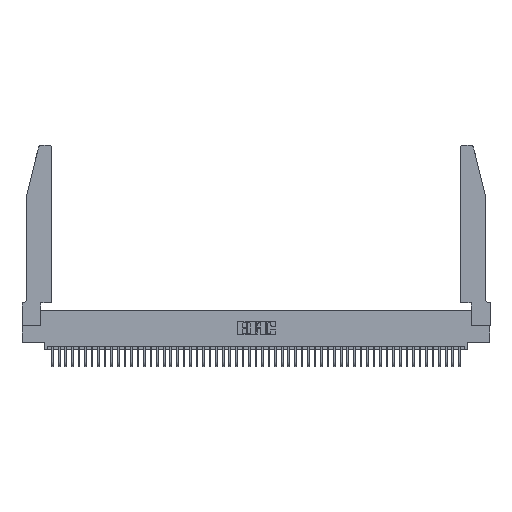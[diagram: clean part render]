
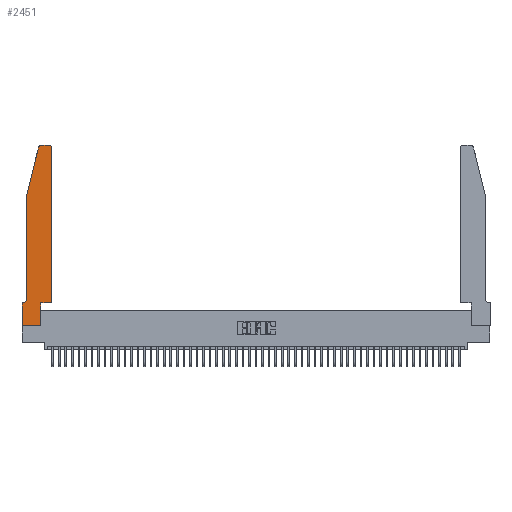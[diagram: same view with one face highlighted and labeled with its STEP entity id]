
A CAD part, top view. The second image highlights one B-rep face of the part: STEP entity #2451.
In plain terms, the highlighted planar face has unit normal (0, 0, 1).
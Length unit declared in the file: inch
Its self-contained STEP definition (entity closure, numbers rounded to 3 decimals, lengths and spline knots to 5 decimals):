
#269 = CARTESIAN_POINT ( 'NONE',  ( 0.0755, 2., 0.37 ) ) ;
#425 = ORIENTED_EDGE ( 'NONE', *, *, #27910, .T. ) ;
#470 = DIRECTION ( 'NONE',  ( 1., 0., 0. ) ) ;
#558 = LINE ( 'NONE', #24356, #9575 ) ;
#656 = EDGE_CURVE ( 'NONE', #18572, #30983, #21931, .T. ) ;
#1385 = DIRECTION ( 'NONE',  ( 0., 1., 0. ) ) ;
#2451 = ADVANCED_FACE ( 'NONE', ( #30536 ), #37271, .T. ) ;
#2888 = DIRECTION ( 'NONE',  ( -1., 0., 0. ) ) ;
#3315 = CARTESIAN_POINT ( 'NONE',  ( 0.2865, 0., 0.37 ) ) ;
#3904 = AXIS2_PLACEMENT_3D ( 'NONE', #21573, #48271, #25416 ) ;
#4101 = CARTESIAN_POINT ( 'NONE',  ( 0.0755, 2., 0.37 ) ) ;
#4486 = EDGE_CURVE ( 'NONE', #43937, #42492, #41733, .T. ) ;
#5169 = CARTESIAN_POINT ( 'NONE',  ( 0.4205, 2.72, 0.37 ) ) ;
#6254 = DIRECTION ( 'NONE',  ( -1., 0., 0. ) ) ;
#6842 = AXIS2_PLACEMENT_3D ( 'NONE', #14297, #18176, #44928 ) ;
#7370 = CARTESIAN_POINT ( 'NONE',  ( 0.25487, 2.72718, 0.37 ) ) ;
#7932 = DIRECTION ( 'NONE',  ( -0.239, -0.971, 0. ) ) ;
#9020 = DIRECTION ( 'NONE',  ( 1., 0., 0. ) ) ;
#9254 = CARTESIAN_POINT ( 'NONE',  ( 0.2865, 0.35, 0.37 ) ) ;
#9575 = VECTOR ( 'NONE', #1385, 39.37008 ) ;
#10505 = LINE ( 'NONE', #15912, #29719 ) ;
#11327 = VECTOR ( 'NONE', #470, 39.37008 ) ;
#12124 = VECTOR ( 'NONE', #2888, 39.37008 ) ;
#13703 = ORIENTED_EDGE ( 'NONE', *, *, #18633, .T. ) ;
#13829 = VECTOR ( 'NONE', #34802, 39.37008 ) ;
#14230 = ORIENTED_EDGE ( 'NONE', *, *, #18502, .T. ) ;
#14297 = CARTESIAN_POINT ( 'NONE',  ( 0., 0.35, 0.37 ) ) ;
#14306 = CIRCLE ( 'NONE', #48393, 0.03 ) ;
#14677 = VERTEX_POINT ( 'NONE', #43139 ) ;
#15912 = CARTESIAN_POINT ( 'NONE',  ( 0.2865, 0.35, 0.37 ) ) ;
#16066 = EDGE_CURVE ( 'NONE', #18029, #41236, #40901, .T. ) ;
#16502 = CARTESIAN_POINT ( 'NONE',  ( 0., 0., 0.37 ) ) ;
#16604 = AXIS2_PLACEMENT_3D ( 'NONE', #44516, #21641, #48350 ) ;
#17129 = ORIENTED_EDGE ( 'NONE', *, *, #16066, .T. ) ;
#17133 = CARTESIAN_POINT ( 'NONE',  ( 0.0055, 0.35, 0.37 ) ) ;
#18029 = VERTEX_POINT ( 'NONE', #43703 ) ;
#18176 = DIRECTION ( 'NONE',  ( 0., 0., 1. ) ) ;
#18502 = EDGE_CURVE ( 'NONE', #46680, #31567, #30557, .T. ) ;
#18572 = VERTEX_POINT ( 'NONE', #23942 ) ;
#18633 = EDGE_CURVE ( 'NONE', #31707, #37220, #14306, .T. ) ;
#19508 = VECTOR ( 'NONE', #7932, 39.37008 ) ;
#20378 = ORIENTED_EDGE ( 'NONE', *, *, #21464, .T. ) ;
#20424 = EDGE_LOOP ( 'NONE', ( #28713, #44259, #20378, #39838, #17129, #42898, #425, #14230, #44186, #38826, #29325, #13703 ) ) ;
#21464 = EDGE_CURVE ( 'NONE', #30983, #14677, #39894, .T. ) ;
#21573 = CARTESIAN_POINT ( 'NONE',  ( 0.284, 2.72, 0.37 ) ) ;
#21641 = DIRECTION ( 'NONE',  ( 0., 0., -1. ) ) ;
#21931 = CIRCLE ( 'NONE', #3904, 0.03 ) ;
#23225 = CARTESIAN_POINT ( 'NONE',  ( 0.4505, 2.72, 0.37 ) ) ;
#23458 = CARTESIAN_POINT ( 'NONE',  ( 0., 0., 0.37 ) ) ;
#23783 = LINE ( 'NONE', #48816, #33989 ) ;
#23942 = CARTESIAN_POINT ( 'NONE',  ( 0.284, 2.75, 0.37 ) ) ;
#24356 = CARTESIAN_POINT ( 'NONE',  ( 0.4505, 0.35, 0.37 ) ) ;
#25416 = DIRECTION ( 'NONE',  ( 1., 0., 0. ) ) ;
#25988 = DIRECTION ( 'NONE',  ( 0., -1., 0. ) ) ;
#26526 = VECTOR ( 'NONE', #6254, 39.37008 ) ;
#27496 = DIRECTION ( 'NONE',  ( 0., 1., 0. ) ) ;
#27910 = EDGE_CURVE ( 'NONE', #41270, #46680, #23783, .T. ) ;
#28713 = ORIENTED_EDGE ( 'NONE', *, *, #41316, .T. ) ;
#29325 = ORIENTED_EDGE ( 'NONE', *, *, #45522, .T. ) ;
#29719 = VECTOR ( 'NONE', #27496, 39.37008 ) ;
#30399 = VECTOR ( 'NONE', #43552, 39.37008 ) ;
#30536 = FACE_OUTER_BOUND ( 'NONE', #20424, .T. ) ;
#30557 = LINE ( 'NONE', #23458, #11327 ) ;
#30862 = EDGE_CURVE ( 'NONE', #41236, #41270, #42679, .T. ) ;
#30983 = VERTEX_POINT ( 'NONE', #7370 ) ;
#31567 = VERTEX_POINT ( 'NONE', #3315 ) ;
#31707 = VERTEX_POINT ( 'NONE', #23225 ) ;
#32008 = DIRECTION ( 'NONE',  ( 0., 0., 1. ) ) ;
#33989 = VECTOR ( 'NONE', #25988, 39.37008 ) ;
#34371 = CARTESIAN_POINT ( 'NONE',  ( 0.4505, 0.35, 0.37 ) ) ;
#34802 = DIRECTION ( 'NONE',  ( 0., -1., 0. ) ) ;
#36422 = CARTESIAN_POINT ( 'NONE',  ( 0., 0.35, 0.37 ) ) ;
#36744 = LINE ( 'NONE', #40574, #26526 ) ;
#37220 = VERTEX_POINT ( 'NONE', #42697 ) ;
#37221 = EDGE_CURVE ( 'NONE', #31567, #43937, #10505, .T. ) ;
#37271 = PLANE ( 'NONE',  #6842 ) ;
#38826 = ORIENTED_EDGE ( 'NONE', *, *, #4486, .T. ) ;
#39838 = ORIENTED_EDGE ( 'NONE', *, *, #42235, .T. ) ;
#39884 = CARTESIAN_POINT ( 'NONE',  ( 0.4505, 0.35, 0.37 ) ) ;
#39894 = LINE ( 'NONE', #4101, #19508 ) ;
#40574 = CARTESIAN_POINT ( 'NONE',  ( 0.2605, 2.75, 0.37 ) ) ;
#40901 = CIRCLE ( 'NONE', #16604, 0.07 ) ;
#41236 = VERTEX_POINT ( 'NONE', #17133 ) ;
#41270 = VERTEX_POINT ( 'NONE', #36422 ) ;
#41316 = EDGE_CURVE ( 'NONE', #37220, #18572, #36744, .T. ) ;
#41733 = LINE ( 'NONE', #39884, #30399 ) ;
#42235 = EDGE_CURVE ( 'NONE', #14677, #18029, #44374, .T. ) ;
#42492 = VERTEX_POINT ( 'NONE', #34371 ) ;
#42679 = LINE ( 'NONE', #48680, #12124 ) ;
#42697 = CARTESIAN_POINT ( 'NONE',  ( 0.4205, 2.75, 0.37 ) ) ;
#42898 = ORIENTED_EDGE ( 'NONE', *, *, #30862, .T. ) ;
#43139 = CARTESIAN_POINT ( 'NONE',  ( 0.0755, 2., 0.37 ) ) ;
#43552 = DIRECTION ( 'NONE',  ( 1., 0., 0. ) ) ;
#43703 = CARTESIAN_POINT ( 'NONE',  ( 0.0755, 0.42, 0.37 ) ) ;
#43937 = VERTEX_POINT ( 'NONE', #9254 ) ;
#44186 = ORIENTED_EDGE ( 'NONE', *, *, #37221, .T. ) ;
#44259 = ORIENTED_EDGE ( 'NONE', *, *, #656, .T. ) ;
#44374 = LINE ( 'NONE', #269, #13829 ) ;
#44516 = CARTESIAN_POINT ( 'NONE',  ( 0.0055, 0.42, 0.37 ) ) ;
#44928 = DIRECTION ( 'NONE',  ( 1., 0., 0. ) ) ;
#45522 = EDGE_CURVE ( 'NONE', #42492, #31707, #558, .T. ) ;
#46680 = VERTEX_POINT ( 'NONE', #16502 ) ;
#48271 = DIRECTION ( 'NONE',  ( 0., 0., 1. ) ) ;
#48350 = DIRECTION ( 'NONE',  ( -1., 0., 0. ) ) ;
#48393 = AXIS2_PLACEMENT_3D ( 'NONE', #5169, #32008, #9020 ) ;
#48680 = CARTESIAN_POINT ( 'NONE',  ( 0.0755, 0.35, 0.37 ) ) ;
#48816 = CARTESIAN_POINT ( 'NONE',  ( 0., 0., 0.37 ) ) ;
